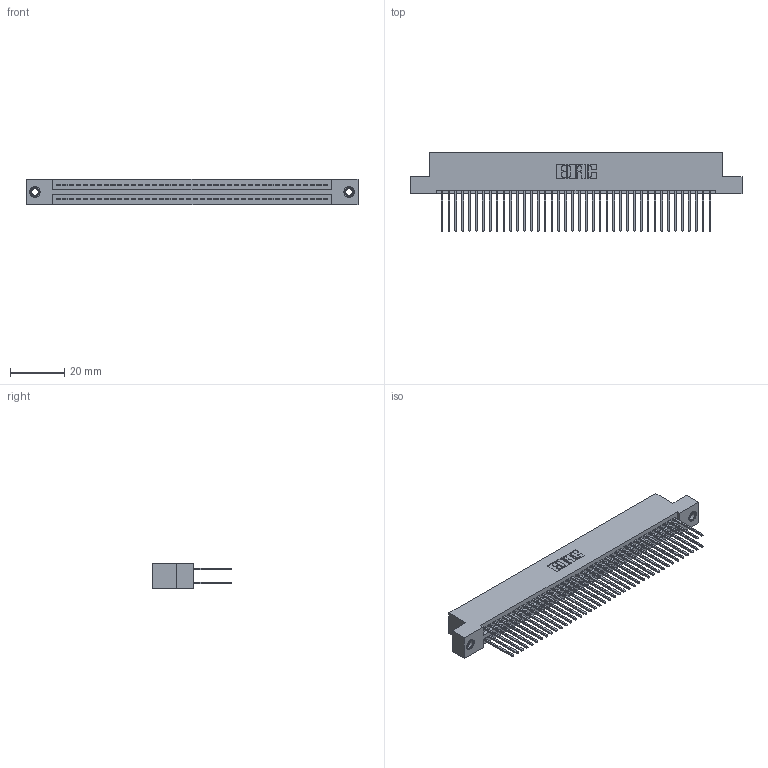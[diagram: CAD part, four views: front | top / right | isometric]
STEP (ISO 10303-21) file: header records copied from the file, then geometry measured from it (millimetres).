
FILE_DESCRIPTION (( 'STEP AP203' ), '1' );
FILE_NAME ('395-080-540-207.STEP', '2018-11-28T03:48:42', ( '' ), ( '' ), 'SwSTEP 2.0', 'SolidWorks 2016', '' );
FILE_SCHEMA (( 'CONFIG_CONTROL_DESIGN' ));
Length unit declared in the file: inch
Products named in the file (4): 395-080-540-207; 345 Part_Flush Mounting Lugs - 0.156 Dia-TI; 345-292-001_345-293-140; 345-250-001_345-250-005-103
Assembly tree (83 placements, depth 2):
  395-080-540-207
    345 Part_Flush Mounting Lugs - 0.156 Dia-TI
    345-292-001_345-293-140  x80
    345-250-001_345-250-005-103  x2
Bounding box: 122.81 x 29.13 x 9.4 mm (x, y, z)
Volume: 12201 mm3; surface area: 19431.3 mm2
Topology: 83 solids, 83 shells, 4186 faces, 12397 edges, 8150 vertices
Faces by surface type: plane 2752, cylinder 1418, cone 12, torus 4
Entity records: 32858 total; most frequent: CARTESIAN_POINT 5491, ORIENTED_EDGE 5418, DIRECTION 4871, EDGE_CURVE 2709, VECTOR 2397, LINE 2397, VERTEX_POINT 1800, AXIS2_PLACEMENT_3D 1237
